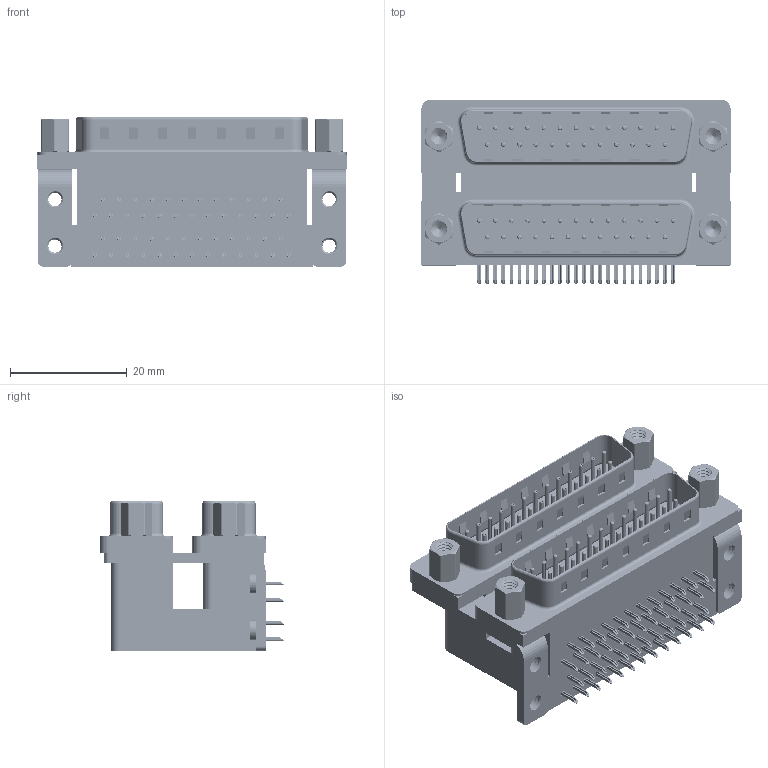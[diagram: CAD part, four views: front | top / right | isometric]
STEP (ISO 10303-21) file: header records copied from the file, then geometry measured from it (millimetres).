
FILE_DESCRIPTION (( 'STEP AP203' ), '1' );
FILE_NAME ('661-025-264-053.STEP', '2020-09-10T23:15:35', ( '' ), ( '' ), 'SwSTEP 2.0', 'SolidWorks 2020', '' );
FILE_SCHEMA (( 'CONFIG_CONTROL_DESIGN' ));
Length unit declared in the file: millimetre
Products named in the file (13): 661 Contact Bottom Upper_L; 661-025-264-053; 661 Contact Bottom Lower; 661 Shell_25 Contacts; 661 4-40 Threaded Board Mount; 661 Contact Top Upper_L; 661 Mounting Bracket_ThruL; 661 Threaded Rivet_4-40; 661 4-40 Hex Standoff 5; 661 Housing Spacer_25 Contacts L; 661 Housing Upper_25 Contacts L; 661 Contact Top Lower; 661 Housing Lower_25 Contacts
Assembly tree (69 placements, depth 2):
  661-025-264-053
    661 Housing Lower_25 Contacts
    661 Housing Spacer_25 Contacts L
    661 Housing Upper_25 Contacts L
    661 Shell_25 Contacts  x2
    661 Contact Bottom Lower  x12
    661 Contact Top Lower  x13
    661 Contact Bottom Upper_L  x12
    661 Contact Top Upper_L  x13
    661 Mounting Bracket_ThruL  x2
    661 4-40 Threaded Board Mount  x4
    661 Threaded Rivet_4-40  x4
    661 4-40 Hex Standoff 5  x4
Bounding box: 53.04 x 31.61 x 25.6 mm (x, y, z)
Volume: 20732 mm3; surface area: 22458.2 mm2
Topology: 69 solids, 69 shells, 5006 faces, 12492 edges, 7754 vertices
Faces by surface type: plane 2994, cylinder 1502, torus 362, cone 100, bspline 48
Entity records: 47458 total; most frequent: CARTESIAN_POINT 12745, ORIENTED_EDGE 6524, DIRECTION 6518, EDGE_CURVE 3262, VECTOR 2364, LINE 2364, VERTEX_POINT 2107, AXIS2_PLACEMENT_3D 2077
